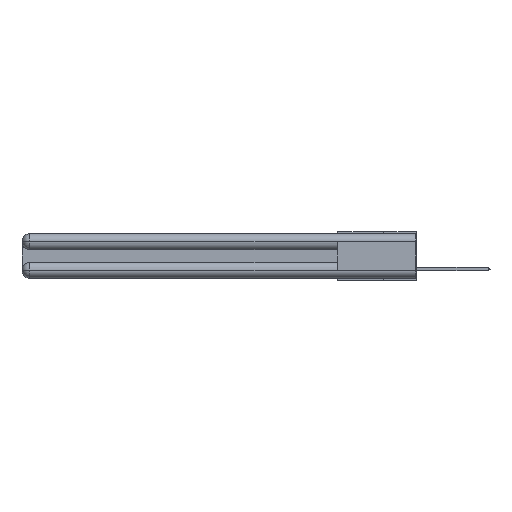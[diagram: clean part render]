
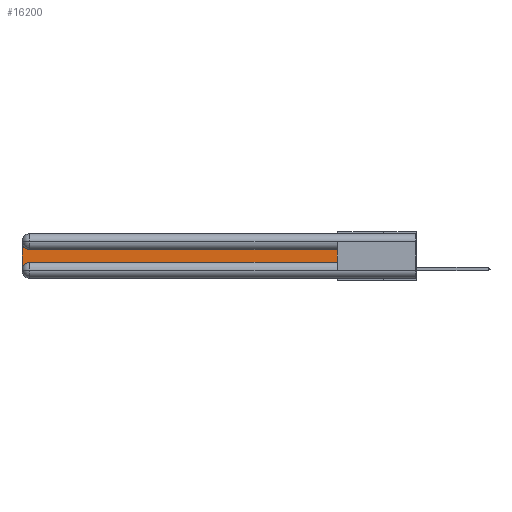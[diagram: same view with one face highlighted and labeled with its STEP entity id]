
A CAD part, left-side view. The second image highlights one B-rep face of the part: STEP entity #16200.
In plain terms, the highlighted planar face has unit normal (-1, 0, 0).
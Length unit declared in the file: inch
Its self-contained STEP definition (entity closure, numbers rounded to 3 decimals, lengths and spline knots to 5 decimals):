
#534 = CARTESIAN_POINT ( 'NONE',  ( 0.075, 3., -0.0625 ) ) ;
#690 = VERTEX_POINT ( 'NONE', #16375 ) ;
#1620 = PLANE ( 'NONE',  #12851 ) ;
#1628 = EDGE_CURVE ( 'NONE', #13668, #10998, #8479, .T. ) ;
#3157 = LINE ( 'NONE', #11139, #6937 ) ;
#3441 = CARTESIAN_POINT ( 'NONE',  ( 0.075, 3., -0.2775 ) ) ;
#3588 = CARTESIAN_POINT ( 'NONE',  ( 0.075, 2.94, -0.2775 ) ) ;
#3697 = DIRECTION ( 'NONE',  ( 0., -1., 0. ) ) ;
#4140 = EDGE_CURVE ( 'NONE', #15155, #690, #10346, .T. ) ;
#4664 = VERTEX_POINT ( 'NONE', #22685 ) ;
#4784 = AXIS2_PLACEMENT_3D ( 'NONE', #3588, #10202, #23193 ) ;
#6016 = CARTESIAN_POINT ( 'NONE',  ( 0.075, 0.6, -0.2175 ) ) ;
#6359 = DIRECTION ( 'NONE',  ( 0., 0., 1. ) ) ;
#6476 = VERTEX_POINT ( 'NONE', #534 ) ;
#6624 = EDGE_LOOP ( 'NONE', ( #15470, #16547, #25194, #8376, #19545, #27431 ) ) ;
#6676 = DIRECTION ( 'NONE',  ( 0., 0., -1. ) ) ;
#6937 = VECTOR ( 'NONE', #6676, 39.37008 ) ;
#7046 = CARTESIAN_POINT ( 'NONE',  ( 0.075, 2.94, -0.0625 ) ) ;
#8376 = ORIENTED_EDGE ( 'NONE', *, *, #4140, .T. ) ;
#8479 = LINE ( 'NONE', #19429, #14656 ) ;
#9565 = EDGE_CURVE ( 'NONE', #690, #13668, #10540, .T. ) ;
#10202 = DIRECTION ( 'NONE',  ( 1., 0., 0. ) ) ;
#10346 = CIRCLE ( 'NONE', #4784, 0.06 ) ;
#10540 = LINE ( 'NONE', #6016, #21123 ) ;
#10998 = VERTEX_POINT ( 'NONE', #13157 ) ;
#11139 = CARTESIAN_POINT ( 'NONE',  ( 0.075, 3., -0.2175 ) ) ;
#11793 = EDGE_CURVE ( 'NONE', #6476, #15155, #3157, .T. ) ;
#12419 = CARTESIAN_POINT ( 'NONE',  ( 0.075, 3., -0.1225 ) ) ;
#12851 = AXIS2_PLACEMENT_3D ( 'NONE', #12419, #14841, #27737 ) ;
#12882 = CARTESIAN_POINT ( 'NONE',  ( 0.075, 0.6, -0.1225 ) ) ;
#13157 = CARTESIAN_POINT ( 'NONE',  ( 0.075, 0.6, -0.1225 ) ) ;
#13539 = DIRECTION ( 'NONE',  ( 0., 0., -1. ) ) ;
#13668 = VERTEX_POINT ( 'NONE', #24225 ) ;
#14503 = LINE ( 'NONE', #12882, #16569 ) ;
#14656 = VECTOR ( 'NONE', #6359, 39.37008 ) ;
#14841 = DIRECTION ( 'NONE',  ( 1., 0., 0. ) ) ;
#15013 = DIRECTION ( 'NONE',  ( 0., 1., 0. ) ) ;
#15155 = VERTEX_POINT ( 'NONE', #3441 ) ;
#15470 = ORIENTED_EDGE ( 'NONE', *, *, #18310, .T. ) ;
#15763 = DIRECTION ( 'NONE',  ( 1., 0., 0. ) ) ;
#16200 = ADVANCED_FACE ( 'NONE', ( #17963 ), #1620, .F. ) ;
#16375 = CARTESIAN_POINT ( 'NONE',  ( 0.075, 2.94, -0.2175 ) ) ;
#16547 = ORIENTED_EDGE ( 'NONE', *, *, #21605, .T. ) ;
#16569 = VECTOR ( 'NONE', #15013, 39.37008 ) ;
#17507 = AXIS2_PLACEMENT_3D ( 'NONE', #7046, #15763, #13539 ) ;
#17963 = FACE_OUTER_BOUND ( 'NONE', #6624, .T. ) ;
#18310 = EDGE_CURVE ( 'NONE', #10998, #4664, #14503, .T. ) ;
#19429 = CARTESIAN_POINT ( 'NONE',  ( 0.075, 0.6, -0.2175 ) ) ;
#19545 = ORIENTED_EDGE ( 'NONE', *, *, #9565, .T. ) ;
#21123 = VECTOR ( 'NONE', #3697, 39.37008 ) ;
#21605 = EDGE_CURVE ( 'NONE', #4664, #6476, #23838, .T. ) ;
#22685 = CARTESIAN_POINT ( 'NONE',  ( 0.075, 2.94, -0.1225 ) ) ;
#23193 = DIRECTION ( 'NONE',  ( 0., 0., -1. ) ) ;
#23838 = CIRCLE ( 'NONE', #17507, 0.06 ) ;
#24225 = CARTESIAN_POINT ( 'NONE',  ( 0.075, 0.6, -0.2175 ) ) ;
#25194 = ORIENTED_EDGE ( 'NONE', *, *, #11793, .T. ) ;
#27431 = ORIENTED_EDGE ( 'NONE', *, *, #1628, .T. ) ;
#27737 = DIRECTION ( 'NONE',  ( 0., 0., -1. ) ) ;
